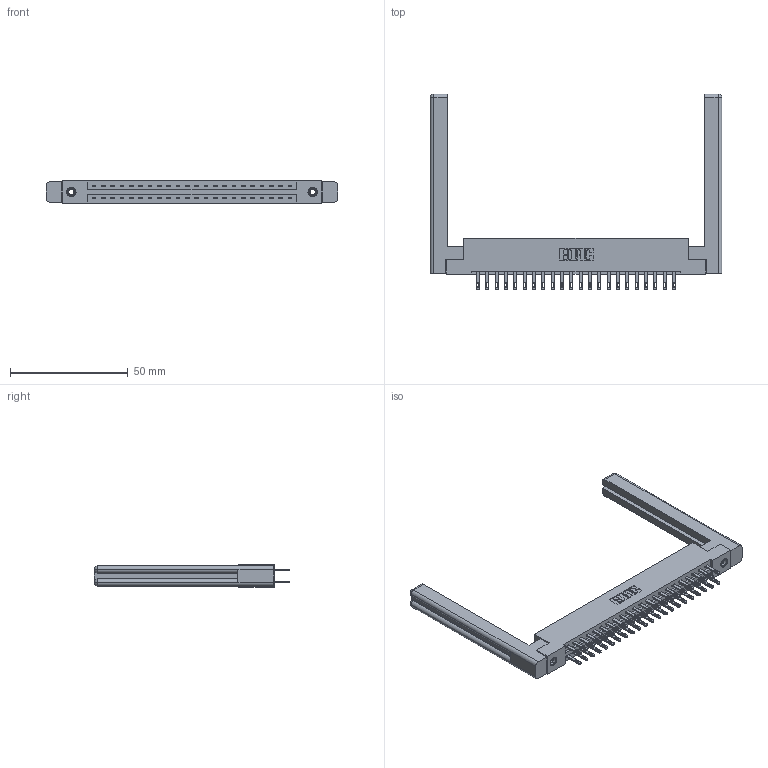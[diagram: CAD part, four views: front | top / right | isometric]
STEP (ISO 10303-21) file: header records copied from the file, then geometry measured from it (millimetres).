
FILE_DESCRIPTION (( 'STEP AP203' ), '1' );
FILE_NAME ('337-044-500-258.STEP', '2019-10-09T12:45:26', ( '' ), ( '' ), 'SwSTEP 2.0', 'SolidWorks 2016', '' );
FILE_SCHEMA (( 'CONFIG_CONTROL_DESIGN' ));
Length unit declared in the file: inch
Products named in the file (5): 345-292-001_345-293-100; 337-044-500-258; 337 Part_Flush Mounting Lugs - 0.156 Dia-TI; 307-220-058; 345-250-001_345-250-001-102
Assembly tree (49 placements, depth 2):
  337-044-500-258
    337 Part_Flush Mounting Lugs - 0.156 Dia-TI
    345-292-001_345-293-100  x44
    345-250-001_345-250-001-102  x2
    307-220-058  x2
Bounding box: 123.8 x 82.94 x 9.4 mm (x, y, z)
Volume: 20057.6 mm3; surface area: 19941.4 mm2
Topology: 49 solids, 49 shells, 2456 faces, 7397 edges, 4918 vertices
Faces by surface type: plane 1562, cylinder 870, cone 12, torus 12
Entity records: 22208 total; most frequent: CARTESIAN_POINT 3765, ORIENTED_EDGE 3640, DIRECTION 3256, EDGE_CURVE 1820, VECTOR 1640, LINE 1640, VERTEX_POINT 1206, AXIS2_PLACEMENT_3D 808
